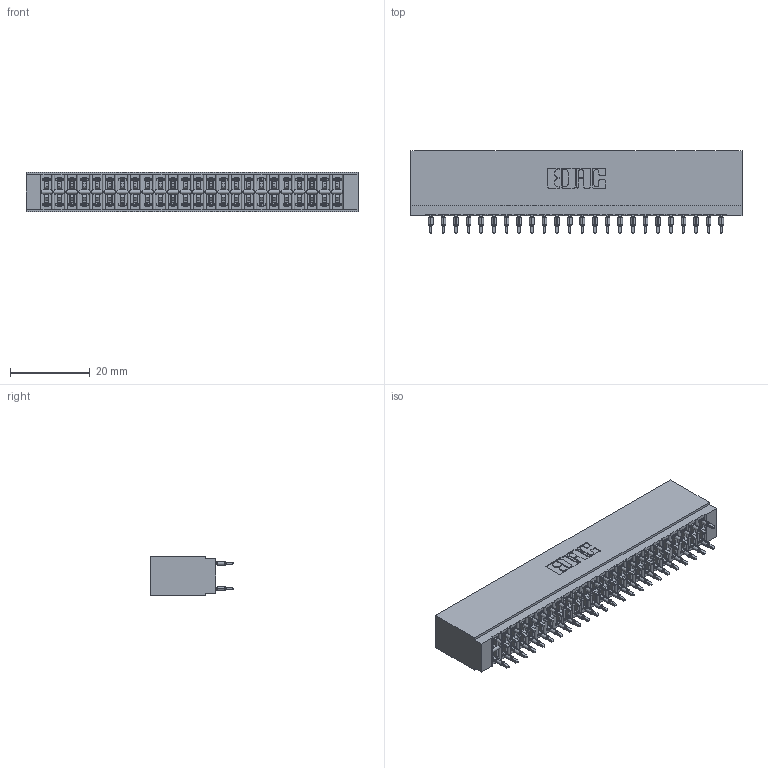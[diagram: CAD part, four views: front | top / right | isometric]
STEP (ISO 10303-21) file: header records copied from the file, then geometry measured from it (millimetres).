
FILE_DESCRIPTION (( 'STEP AP203' ), '1' );
FILE_NAME ('746-048-560-201.STEP', '2026-02-27T18:37:16', ( '' ), ( '' ), 'SwSTEP 2.0', 'SolidWorks 2023', '' );
FILE_SCHEMA (( 'CONFIG_CONTROL_DESIGN' ));
Length unit declared in the file: millimetre
Products named in the file (3): 746 Part_.515 Slot Depth - 01; 746-292-001_560; 746-048-560-201
Assembly tree (49 placements, depth 2):
  746-048-560-201
    746 Part_.515 Slot Depth - 01
    746-292-001_560  x48
Bounding box: 83.44 x 20.82 x 9.91 mm (x, y, z)
Volume: 9225.9 mm3; surface area: 15236.3 mm2
Topology: 49 solids, 49 shells, 4633 faces, 12887 edges, 8263 vertices
Faces by surface type: plane 2311, cylinder 1074, bspline 960, torus 288
Entity records: 39764 total; most frequent: CARTESIAN_POINT 8059, ORIENTED_EDGE 6786, DIRECTION 5703, EDGE_CURVE 3393, LINE 2961, VECTOR 2961, VERTEX_POINT 2247, AXIS2_PLACEMENT_3D 1371
